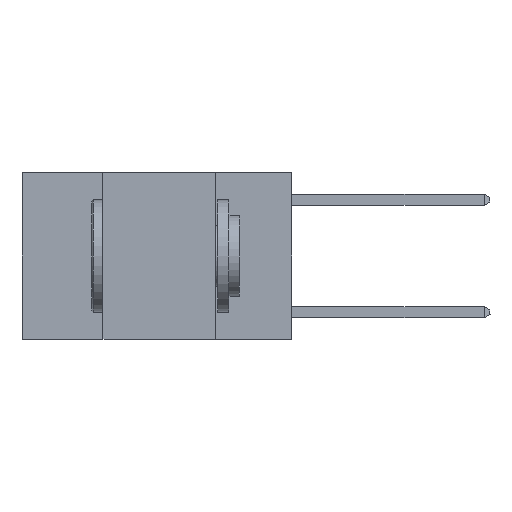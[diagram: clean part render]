
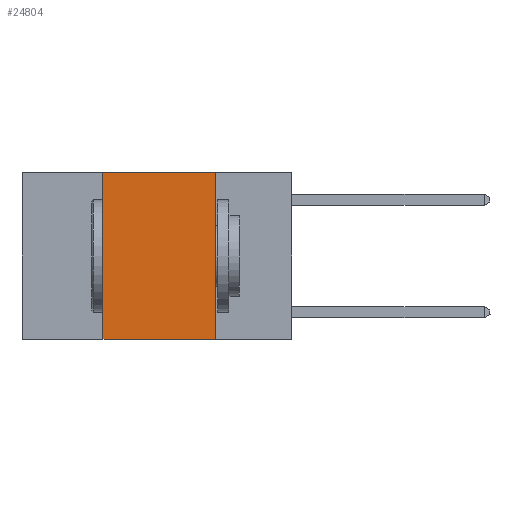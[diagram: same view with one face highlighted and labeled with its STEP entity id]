
A CAD part, left-side view. The second image highlights one B-rep face of the part: STEP entity #24804.
In plain terms, the highlighted planar face has unit normal (-1, 0, 0).
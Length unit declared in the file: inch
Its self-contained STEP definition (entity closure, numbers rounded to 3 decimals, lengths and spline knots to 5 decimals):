
#991 = ORIENTED_EDGE ( 'NONE', *, *, #14149, .F. ) ;
#2505 = ORIENTED_EDGE ( 'NONE', *, *, #27038, .T. ) ;
#3127 = CARTESIAN_POINT ( 'NONE',  ( 0., 0.6, 0. ) ) ;
#4480 = CARTESIAN_POINT ( 'NONE',  ( 0., 0.17, 0. ) ) ;
#5040 = DIRECTION ( 'NONE',  ( 0., 0., 1. ) ) ;
#5172 = CARTESIAN_POINT ( 'NONE',  ( 0., 0.42, 0. ) ) ;
#5634 = CARTESIAN_POINT ( 'NONE',  ( 0., 0.6, 0. ) ) ;
#6022 = EDGE_LOOP ( 'NONE', ( #20231, #17003, #991, #2505 ) ) ;
#7191 = DIRECTION ( 'NONE',  ( 0., -1., 0. ) ) ;
#8519 = FACE_OUTER_BOUND ( 'NONE', #6022, .T. ) ;
#9594 = VECTOR ( 'NONE', #15838, 39.37008 ) ;
#10561 = VERTEX_POINT ( 'NONE', #15320 ) ;
#10866 = AXIS2_PLACEMENT_3D ( 'NONE', #3127, #22075, #11510 ) ;
#11305 = CARTESIAN_POINT ( 'NONE',  ( 0., 0.6, -0.37 ) ) ;
#11510 = DIRECTION ( 'NONE',  ( 0., 0., -1. ) ) ;
#11696 = VERTEX_POINT ( 'NONE', #20140 ) ;
#12102 = VECTOR ( 'NONE', #13154, 39.37008 ) ;
#13154 = DIRECTION ( 'NONE',  ( 0., 0., -1. ) ) ;
#13567 = VERTEX_POINT ( 'NONE', #18473 ) ;
#14149 = EDGE_CURVE ( 'NONE', #13567, #11696, #23710, .T. ) ;
#15320 = CARTESIAN_POINT ( 'NONE',  ( 0., 0.17, 0. ) ) ;
#15343 = CARTESIAN_POINT ( 'NONE',  ( 0., 0.17, -0.37 ) ) ;
#15838 = DIRECTION ( 'NONE',  ( 0., -1., 0. ) ) ;
#15968 = LINE ( 'NONE', #5634, #9594 ) ;
#17003 = ORIENTED_EDGE ( 'NONE', *, *, #25817, .F. ) ;
#17465 = VERTEX_POINT ( 'NONE', #15343 ) ;
#17550 = VECTOR ( 'NONE', #7191, 39.37008 ) ;
#18473 = CARTESIAN_POINT ( 'NONE',  ( 0., 0.42, -0.37 ) ) ;
#20140 = CARTESIAN_POINT ( 'NONE',  ( 0., 0.42, 0. ) ) ;
#20231 = ORIENTED_EDGE ( 'NONE', *, *, #21017, .F. ) ;
#21017 = EDGE_CURVE ( 'NONE', #10561, #17465, #25065, .T. ) ;
#22075 = DIRECTION ( 'NONE',  ( 1., 0., 0. ) ) ;
#23710 = LINE ( 'NONE', #5172, #26176 ) ;
#24328 = LINE ( 'NONE', #11305, #17550 ) ;
#24804 = ADVANCED_FACE ( 'NONE', ( #8519 ), #26178, .F. ) ;
#25065 = LINE ( 'NONE', #4480, #12102 ) ;
#25817 = EDGE_CURVE ( 'NONE', #11696, #10561, #15968, .T. ) ;
#26176 = VECTOR ( 'NONE', #5040, 39.37008 ) ;
#26178 = PLANE ( 'NONE',  #10866 ) ;
#27038 = EDGE_CURVE ( 'NONE', #13567, #17465, #24328, .T. ) ;
